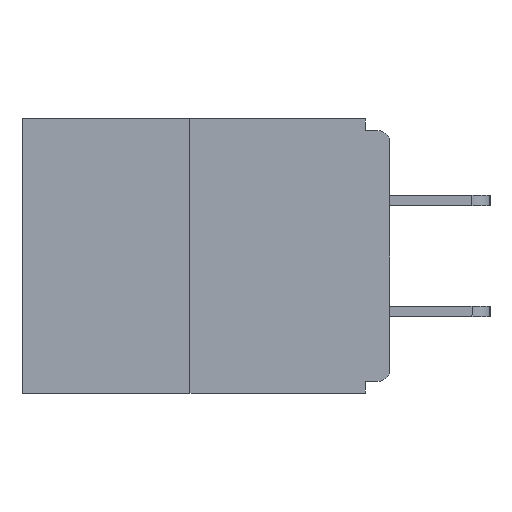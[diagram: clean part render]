
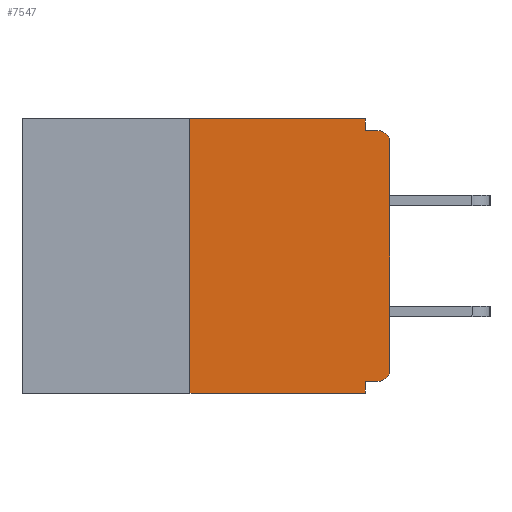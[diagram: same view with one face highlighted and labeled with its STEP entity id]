
A CAD part, left-side view. The second image highlights one B-rep face of the part: STEP entity #7547.
In plain terms, the highlighted planar face has unit normal (-1, 0, 0).
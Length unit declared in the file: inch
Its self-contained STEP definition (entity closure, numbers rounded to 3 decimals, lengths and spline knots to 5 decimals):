
#125 = ORIENTED_EDGE ( 'NONE', *, *, #4769, .T. ) ;
#148 = LINE ( 'NONE', #2205, #1853 ) ;
#157 = VECTOR ( 'NONE', #1647, 39.37008 ) ;
#290 = VERTEX_POINT ( 'NONE', #6857 ) ;
#320 = CARTESIAN_POINT ( 'NONE',  ( 0., 0.015, -0.03 ) ) ;
#394 = VECTOR ( 'NONE', #1555, 39.37008 ) ;
#623 = ORIENTED_EDGE ( 'NONE', *, *, #3055, .T. ) ;
#1106 = ORIENTED_EDGE ( 'NONE', *, *, #1614, .T. ) ;
#1522 = EDGE_CURVE ( 'NONE', #9996, #6961, #10649, .T. ) ;
#1555 = DIRECTION ( 'NONE',  ( 0., 0., 1. ) ) ;
#1614 = EDGE_CURVE ( 'NONE', #10759, #290, #6732, .T. ) ;
#1616 = DIRECTION ( 'NONE',  ( 0., -1., 0. ) ) ;
#1629 = CARTESIAN_POINT ( 'NONE',  ( 0., 0., -0.328 ) ) ;
#1647 = DIRECTION ( 'NONE',  ( 0., -1., 0. ) ) ;
#1853 = VECTOR ( 'NONE', #7711, 39.37008 ) ;
#1933 = LINE ( 'NONE', #9062, #5620 ) ;
#2205 = CARTESIAN_POINT ( 'NONE',  ( 0., 0.031, -0.343 ) ) ;
#2314 = CARTESIAN_POINT ( 'NONE',  ( 0., 0.25, -0.343 ) ) ;
#2440 = AXIS2_PLACEMENT_3D ( 'NONE', #320, #9456, #8460 ) ;
#2646 = EDGE_CURVE ( 'NONE', #3518, #290, #148, .T. ) ;
#3055 = EDGE_CURVE ( 'NONE', #8938, #7651, #3671, .T. ) ;
#3200 = ORIENTED_EDGE ( 'NONE', *, *, #7733, .T. ) ;
#3514 = DIRECTION ( 'NONE',  ( 0., -1., 0. ) ) ;
#3518 = VERTEX_POINT ( 'NONE', #11263 ) ;
#3640 = AXIS2_PLACEMENT_3D ( 'NONE', #9174, #3756, #5588 ) ;
#3671 = CIRCLE ( 'NONE', #8742, 0.015 ) ;
#3733 = DIRECTION ( 'NONE',  ( -1., 0., 0. ) ) ;
#3756 = DIRECTION ( 'NONE',  ( 1., 0., 0. ) ) ;
#3849 = CARTESIAN_POINT ( 'NONE',  ( 0., 0.25, 0. ) ) ;
#3866 = VERTEX_POINT ( 'NONE', #10451 ) ;
#4404 = FACE_OUTER_BOUND ( 'NONE', #9539, .T. ) ;
#4525 = ORIENTED_EDGE ( 'NONE', *, *, #6152, .F. ) ;
#4690 = DIRECTION ( 'NONE',  ( 0., 0., 1. ) ) ;
#4718 = PLANE ( 'NONE',  #3640 ) ;
#4769 = EDGE_CURVE ( 'NONE', #7651, #9618, #11159, .T. ) ;
#4815 = CARTESIAN_POINT ( 'NONE',  ( 0., 0.25, 0. ) ) ;
#4897 = EDGE_CURVE ( 'NONE', #3866, #9513, #1933, .T. ) ;
#5349 = CARTESIAN_POINT ( 'NONE',  ( 0., 0.015, -0.015 ) ) ;
#5355 = ORIENTED_EDGE ( 'NONE', *, *, #4897, .F. ) ;
#5397 = CIRCLE ( 'NONE', #2440, 0.015 ) ;
#5527 = EDGE_CURVE ( 'NONE', #6961, #3866, #7493, .T. ) ;
#5588 = DIRECTION ( 'NONE',  ( 0., 0., -1. ) ) ;
#5620 = VECTOR ( 'NONE', #3514, 39.37008 ) ;
#5710 = VECTOR ( 'NONE', #4690, 39.37008 ) ;
#6152 = EDGE_CURVE ( 'NONE', #10759, #9996, #10804, .T. ) ;
#6438 = CARTESIAN_POINT ( 'NONE',  ( 0., 0., -0.313 ) ) ;
#6490 = CARTESIAN_POINT ( 'NONE',  ( 0., 0.015, -0.313 ) ) ;
#6609 = DIRECTION ( 'NONE',  ( 0., 0., -1. ) ) ;
#6732 = LINE ( 'NONE', #11702, #157 ) ;
#6857 = CARTESIAN_POINT ( 'NONE',  ( 0., 0.031, -0.343 ) ) ;
#6961 = VERTEX_POINT ( 'NONE', #9448 ) ;
#7470 = ORIENTED_EDGE ( 'NONE', *, *, #2646, .F. ) ;
#7493 = LINE ( 'NONE', #9520, #10705 ) ;
#7536 = VECTOR ( 'NONE', #8008, 39.37008 ) ;
#7547 = ADVANCED_FACE ( 'NONE', ( #4404 ), #4718, .F. ) ;
#7651 = VERTEX_POINT ( 'NONE', #6438 ) ;
#7709 = VECTOR ( 'NONE', #1616, 39.37008 ) ;
#7711 = DIRECTION ( 'NONE',  ( 0., 0., -1. ) ) ;
#7733 = EDGE_CURVE ( 'NONE', #9618, #9513, #5397, .T. ) ;
#7734 = CARTESIAN_POINT ( 'NONE',  ( 0., 0.015, -0.328 ) ) ;
#8008 = DIRECTION ( 'NONE',  ( 0., 1., 0. ) ) ;
#8460 = DIRECTION ( 'NONE',  ( 0., 0., -1. ) ) ;
#8695 = EDGE_CURVE ( 'NONE', #8938, #3518, #8941, .T. ) ;
#8742 = AXIS2_PLACEMENT_3D ( 'NONE', #6490, #3733, #6609 ) ;
#8799 = CARTESIAN_POINT ( 'NONE',  ( 0., 0., 0. ) ) ;
#8938 = VERTEX_POINT ( 'NONE', #7734 ) ;
#8941 = LINE ( 'NONE', #1629, #7536 ) ;
#9062 = CARTESIAN_POINT ( 'NONE',  ( 0., 0., -0.015 ) ) ;
#9165 = CARTESIAN_POINT ( 'NONE',  ( 0., 0., -0.03 ) ) ;
#9174 = CARTESIAN_POINT ( 'NONE',  ( 0., 0.46, 0. ) ) ;
#9448 = CARTESIAN_POINT ( 'NONE',  ( 0., 0.031, 0. ) ) ;
#9456 = DIRECTION ( 'NONE',  ( -1., 0., 0. ) ) ;
#9513 = VERTEX_POINT ( 'NONE', #5349 ) ;
#9520 = CARTESIAN_POINT ( 'NONE',  ( 0., 0.031, 0. ) ) ;
#9539 = EDGE_LOOP ( 'NONE', ( #10424, #4525, #1106, #7470, #10920, #623, #125, #3200, #5355, #10477 ) ) ;
#9618 = VERTEX_POINT ( 'NONE', #9165 ) ;
#9996 = VERTEX_POINT ( 'NONE', #3849 ) ;
#10424 = ORIENTED_EDGE ( 'NONE', *, *, #1522, .F. ) ;
#10451 = CARTESIAN_POINT ( 'NONE',  ( 0., 0.031, -0.015 ) ) ;
#10477 = ORIENTED_EDGE ( 'NONE', *, *, #5527, .F. ) ;
#10649 = LINE ( 'NONE', #10800, #7709 ) ;
#10705 = VECTOR ( 'NONE', #11279, 39.37008 ) ;
#10759 = VERTEX_POINT ( 'NONE', #2314 ) ;
#10800 = CARTESIAN_POINT ( 'NONE',  ( 0., 0.46, 0. ) ) ;
#10804 = LINE ( 'NONE', #4815, #5710 ) ;
#10920 = ORIENTED_EDGE ( 'NONE', *, *, #8695, .F. ) ;
#11159 = LINE ( 'NONE', #8799, #394 ) ;
#11263 = CARTESIAN_POINT ( 'NONE',  ( 0., 0.031, -0.328 ) ) ;
#11279 = DIRECTION ( 'NONE',  ( 0., 0., -1. ) ) ;
#11702 = CARTESIAN_POINT ( 'NONE',  ( 0., 0.46, -0.343 ) ) ;
